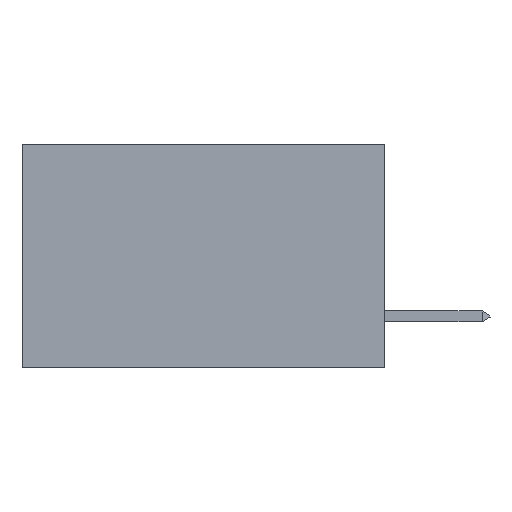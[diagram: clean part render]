
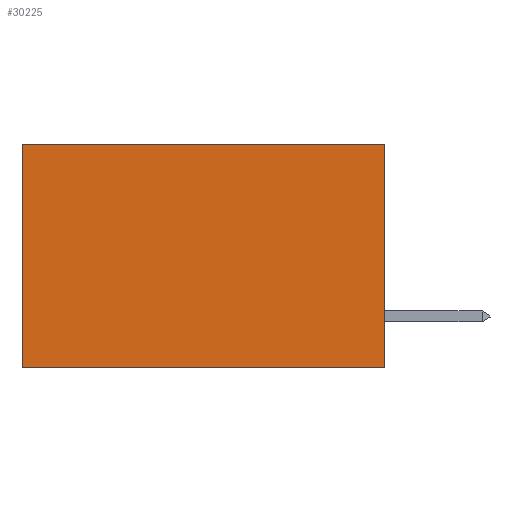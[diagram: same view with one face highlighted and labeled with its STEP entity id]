
A CAD part, left-side view. The second image highlights one B-rep face of the part: STEP entity #30225.
In plain terms, the highlighted planar face has unit normal (-1, 0, 0).
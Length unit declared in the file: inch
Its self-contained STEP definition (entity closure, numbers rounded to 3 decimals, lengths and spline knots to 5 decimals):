
#909 = DIRECTION ( 'NONE',  ( 0., 0., -1. ) ) ;
#1228 = DIRECTION ( 'NONE',  ( 0., 0., -1. ) ) ;
#1421 = CARTESIAN_POINT ( 'NONE',  ( 0.2875, 0.6, 0. ) ) ;
#1722 = VECTOR ( 'NONE', #17294, 39.37008 ) ;
#2404 = VERTEX_POINT ( 'NONE', #28129 ) ;
#3734 = EDGE_CURVE ( 'NONE', #22349, #2404, #30972, .T. ) ;
#5133 = PLANE ( 'NONE',  #19187 ) ;
#7300 = CARTESIAN_POINT ( 'NONE',  ( 0.2875, 0., 0. ) ) ;
#8273 = ORIENTED_EDGE ( 'NONE', *, *, #17891, .T. ) ;
#10367 = DIRECTION ( 'NONE',  ( 1., 0., 0. ) ) ;
#13234 = DIRECTION ( 'NONE',  ( 0., 0., -1. ) ) ;
#14699 = CARTESIAN_POINT ( 'NONE',  ( 0.2875, 0., 0. ) ) ;
#16499 = CARTESIAN_POINT ( 'NONE',  ( 0.2875, 0.6, 0. ) ) ;
#17294 = DIRECTION ( 'NONE',  ( 0., 1., 0. ) ) ;
#17747 = ORIENTED_EDGE ( 'NONE', *, *, #3734, .T. ) ;
#17785 = CARTESIAN_POINT ( 'NONE',  ( 0.2875, 0., -0.37 ) ) ;
#17891 = EDGE_CURVE ( 'NONE', #32043, #22349, #20571, .T. ) ;
#18096 = VECTOR ( 'NONE', #1228, 39.37008 ) ;
#18860 = LINE ( 'NONE', #7300, #20082 ) ;
#19187 = AXIS2_PLACEMENT_3D ( 'NONE', #29989, #10367, #909 ) ;
#19614 = EDGE_CURVE ( 'NONE', #32043, #26982, #18860, .T. ) ;
#19833 = FACE_OUTER_BOUND ( 'NONE', #23372, .T. ) ;
#20082 = VECTOR ( 'NONE', #13234, 39.37008 ) ;
#20571 = LINE ( 'NONE', #29926, #1722 ) ;
#20652 = EDGE_CURVE ( 'NONE', #26982, #2404, #33316, .T. ) ;
#22349 = VERTEX_POINT ( 'NONE', #1421 ) ;
#22949 = ORIENTED_EDGE ( 'NONE', *, *, #19614, .F. ) ;
#23372 = EDGE_LOOP ( 'NONE', ( #17747, #24374, #22949, #8273 ) ) ;
#24374 = ORIENTED_EDGE ( 'NONE', *, *, #20652, .F. ) ;
#26462 = VECTOR ( 'NONE', #32231, 39.37008 ) ;
#26982 = VERTEX_POINT ( 'NONE', #17785 ) ;
#28129 = CARTESIAN_POINT ( 'NONE',  ( 0.2875, 0.6, -0.37 ) ) ;
#29683 = CARTESIAN_POINT ( 'NONE',  ( 0.2875, 0., -0.37 ) ) ;
#29926 = CARTESIAN_POINT ( 'NONE',  ( 0.2875, 0., 0. ) ) ;
#29989 = CARTESIAN_POINT ( 'NONE',  ( 0.2875, 0., 0. ) ) ;
#30225 = ADVANCED_FACE ( 'NONE', ( #19833 ), #5133, .F. ) ;
#30972 = LINE ( 'NONE', #16499, #18096 ) ;
#32043 = VERTEX_POINT ( 'NONE', #14699 ) ;
#32231 = DIRECTION ( 'NONE',  ( 0., 1., 0. ) ) ;
#33316 = LINE ( 'NONE', #29683, #26462 ) ;
